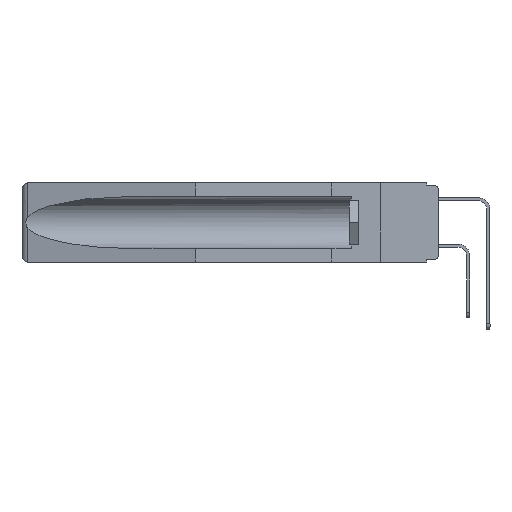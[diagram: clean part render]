
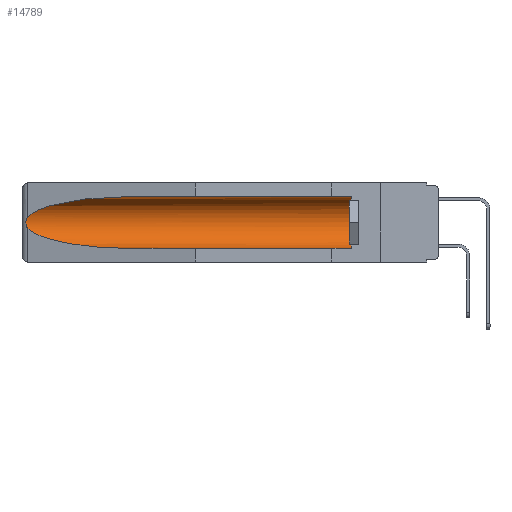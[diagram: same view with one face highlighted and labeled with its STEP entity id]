
A CAD part, left-side view. The second image highlights one B-rep face of the part: STEP entity #14789.
In plain terms, the highlighted cylindrical face has radius 2.857 mm (diameter 5.715 mm), a partial arc.
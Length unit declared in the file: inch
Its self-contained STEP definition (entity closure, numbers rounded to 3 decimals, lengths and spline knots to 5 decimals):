
#332 = CARTESIAN_POINT ( 'NONE',  ( 0.155, -0.30754, -0.284 ) ) ;
#1160 = EDGE_LOOP ( 'NONE', ( #1386, #6768, #13357, #7508, #3260, #12923 ) ) ;
#1243 = CARTESIAN_POINT ( 'NONE',  ( 0.2675, 1.53308, -0.17534 ) ) ;
#1386 = ORIENTED_EDGE ( 'NONE', *, *, #13683, .T. ) ;
#1438 = CARTESIAN_POINT ( 'NONE',  ( 0.155, 1.07973, -0.284 ) ) ;
#2677 = CARTESIAN_POINT ( 'NONE',  ( 0.25451, 1.48313, -0.24835 ) ) ;
#2889 = CARTESIAN_POINT ( 'NONE',  ( 0.26537, 1.52718, -0.19328 ) ) ;
#2916 = EDGE_CURVE ( 'NONE', #11876, #12618, #5496, .T. ) ;
#3066 =( BOUNDED_CURVE ( )  B_SPLINE_CURVE ( 3, ( #2889, #2677, #15294, #7375 ),
 .UNSPECIFIED., .F., .T. ) 
 B_SPLINE_CURVE_WITH_KNOTS ( ( 4, 4 ),
 ( 0.1948, 1.5708 ),
 .UNSPECIFIED. ) 
 CURVE ( )  GEOMETRIC_REPRESENTATION_ITEM ( )  RATIONAL_B_SPLINE_CURVE ( ( 1., 0.848, 0.848, 1. ) ) 
 REPRESENTATION_ITEM ( '' )  );
#3180 = VERTEX_POINT ( 'NONE', #14767 ) ;
#3260 = ORIENTED_EDGE ( 'NONE', *, *, #2916, .T. ) ;
#3418 = EDGE_CURVE ( 'NONE', #11876, #7869, #19400, .T. ) ;
#4147 = CARTESIAN_POINT ( 'NONE',  ( 0.26597, 1.5296, -0.19026 ) ) ;
#4263 = EDGE_CURVE ( 'NONE', #7917, #7869, #3066, .T. ) ;
#4789 = CARTESIAN_POINT ( 'NONE',  ( 0.155, -0.30754, -0.059 ) ) ;
#4934 = VECTOR ( 'NONE', #11145, 39.37008 ) ;
#5496 = CIRCLE ( 'NONE', #14162, 0.1125 ) ;
#5531 = CARTESIAN_POINT ( 'NONE',  ( 0.155, -0.30754, -0.1715 ) ) ;
#5630 = CYLINDRICAL_SURFACE ( 'NONE', #15392, 0.1125 ) ;
#5997 = CARTESIAN_POINT ( 'NONE',  ( 0.2675, 1.53308, -0.16763 ) ) ;
#6028 = EDGE_CURVE ( 'NONE', #12618, #3180, #13093, .T. ) ;
#6768 = ORIENTED_EDGE ( 'NONE', *, *, #10613, .T. ) ;
#7107 = DIRECTION ( 'NONE',  ( 0., 0., 1. ) ) ;
#7319 =( BOUNDED_CURVE ( )  B_SPLINE_CURVE ( 3, ( #12797, #11233, #14150, #19040 ),
 .UNSPECIFIED., .F., .F. ) 
 B_SPLINE_CURVE_WITH_KNOTS ( ( 4, 4 ),
 ( 4.71239, 6.08839 ),
 .UNSPECIFIED. ) 
 CURVE ( )  GEOMETRIC_REPRESENTATION_ITEM ( )  RATIONAL_B_SPLINE_CURVE ( ( 1., 0.848, 0.848, 1. ) ) 
 REPRESENTATION_ITEM ( '' )  );
#7375 = CARTESIAN_POINT ( 'NONE',  ( 0.155, 1.07973, -0.284 ) ) ;
#7382 = CARTESIAN_POINT ( 'NONE',  ( 0.26537, 1.52718, -0.19328 ) ) ;
#7508 = ORIENTED_EDGE ( 'NONE', *, *, #3418, .F. ) ;
#7869 = VERTEX_POINT ( 'NONE', #1438 ) ;
#7917 = VERTEX_POINT ( 'NONE', #19239 ) ;
#9051 = B_SPLINE_CURVE_WITH_KNOTS ( 'NONE', 3,
 ( #17070, #18542, #12083, #12386, #5997, #1243, #20099, #16870, #4147, #7382 ),
 .UNSPECIFIED., .F., .F.,
 ( 4, 2, 2, 2, 4 ),
 ( 0., 0.00029, 0.00058, 0.00087, 0.00117 ),
 .UNSPECIFIED. ) ;
#9807 = CARTESIAN_POINT ( 'NONE',  ( 0.26537, 1.52718, -0.14972 ) ) ;
#10613 = EDGE_CURVE ( 'NONE', #17772, #7917, #9051, .T. ) ;
#10702 = DIRECTION ( 'NONE',  ( 0., -1., 0. ) ) ;
#11145 = DIRECTION ( 'NONE',  ( 0., 1., 0. ) ) ;
#11233 = CARTESIAN_POINT ( 'NONE',  ( 0.21114, 1.30732, -0.059 ) ) ;
#11373 = DIRECTION ( 'NONE',  ( 0., 1., 0. ) ) ;
#11876 = VERTEX_POINT ( 'NONE', #13160 ) ;
#12083 = CARTESIAN_POINT ( 'NONE',  ( 0.26654, 1.53092, -0.15636 ) ) ;
#12168 = CARTESIAN_POINT ( 'NONE',  ( 0.155, 0.126, -0.1715 ) ) ;
#12386 = CARTESIAN_POINT ( 'NONE',  ( 0.2673, 1.5327, -0.16383 ) ) ;
#12618 = VERTEX_POINT ( 'NONE', #12784 ) ;
#12784 = CARTESIAN_POINT ( 'NONE',  ( 0.155, 0.126, -0.059 ) ) ;
#12797 = CARTESIAN_POINT ( 'NONE',  ( 0.155, 1.07973, -0.059 ) ) ;
#12923 = ORIENTED_EDGE ( 'NONE', *, *, #6028, .T. ) ;
#13093 = LINE ( 'NONE', #4789, #4934 ) ;
#13160 = CARTESIAN_POINT ( 'NONE',  ( 0.155, 0.126, -0.284 ) ) ;
#13161 = FACE_OUTER_BOUND ( 'NONE', #1160, .T. ) ;
#13357 = ORIENTED_EDGE ( 'NONE', *, *, #4263, .T. ) ;
#13683 = EDGE_CURVE ( 'NONE', #3180, #17772, #7319, .T. ) ;
#14150 = CARTESIAN_POINT ( 'NONE',  ( 0.25451, 1.48313, -0.09465 ) ) ;
#14162 = AXIS2_PLACEMENT_3D ( 'NONE', #12168, #10702, #17059 ) ;
#14767 = CARTESIAN_POINT ( 'NONE',  ( 0.155, 1.07973, -0.059 ) ) ;
#14789 = ADVANCED_FACE ( 'NONE', ( #13161 ), #5630, .F. ) ;
#15294 = CARTESIAN_POINT ( 'NONE',  ( 0.21114, 1.30732, -0.284 ) ) ;
#15392 = AXIS2_PLACEMENT_3D ( 'NONE', #5531, #16798, #7107 ) ;
#16179 = VECTOR ( 'NONE', #11373, 39.37008 ) ;
#16798 = DIRECTION ( 'NONE',  ( 0., 1., 0. ) ) ;
#16870 = CARTESIAN_POINT ( 'NONE',  ( 0.26655, 1.53094, -0.18657 ) ) ;
#17059 = DIRECTION ( 'NONE',  ( 0., 0., 1. ) ) ;
#17070 = CARTESIAN_POINT ( 'NONE',  ( 0.26537, 1.52718, -0.14972 ) ) ;
#17772 = VERTEX_POINT ( 'NONE', #9807 ) ;
#18542 = CARTESIAN_POINT ( 'NONE',  ( 0.26597, 1.52961, -0.15275 ) ) ;
#19040 = CARTESIAN_POINT ( 'NONE',  ( 0.26537, 1.52718, -0.14972 ) ) ;
#19239 = CARTESIAN_POINT ( 'NONE',  ( 0.26537, 1.52718, -0.19328 ) ) ;
#19400 = LINE ( 'NONE', #332, #16179 ) ;
#20099 = CARTESIAN_POINT ( 'NONE',  ( 0.2673, 1.53269, -0.17917 ) ) ;
